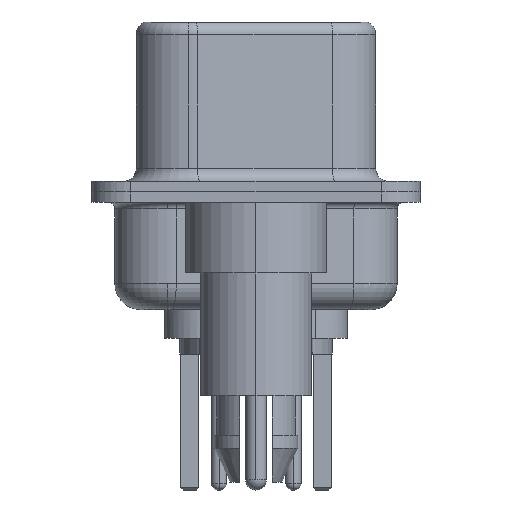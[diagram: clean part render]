
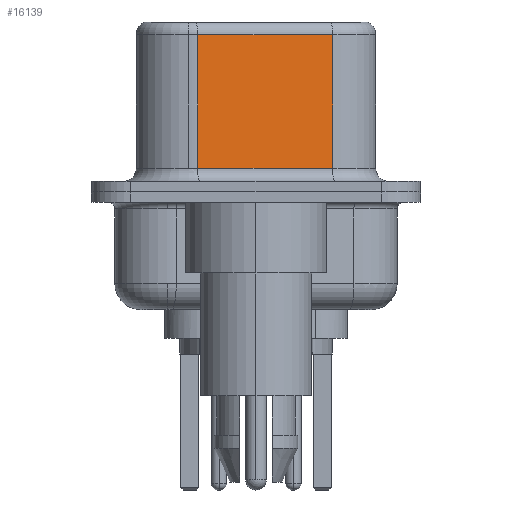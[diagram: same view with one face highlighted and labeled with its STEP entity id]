
A CAD part, left-side view. The second image highlights one B-rep face of the part: STEP entity #16139.
In plain terms, the highlighted planar face has unit normal (-0.985, -0.174, 0).
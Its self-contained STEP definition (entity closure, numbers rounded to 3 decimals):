
#51 = CARTESIAN_POINT ( 'NONE',  ( 4.58, -2.927, 6.02 ) ) ;
#411 = AXIS2_PLACEMENT_3D ( 'NONE', #12200, #4198, #13582 ) ;
#556 = VECTOR ( 'NONE', #16919, 1000. ) ;
#986 = CARTESIAN_POINT ( 'NONE',  ( 3.67, 2.233, 6.02 ) ) ;
#1496 = ORIENTED_EDGE ( 'NONE', *, *, #4866, .T. ) ;
#2880 = PLANE ( 'NONE',  #411 ) ;
#3615 = FACE_OUTER_BOUND ( 'NONE', #12085, .T. ) ;
#3982 = CARTESIAN_POINT ( 'NONE',  ( 3.67, 2.233, 6.52 ) ) ;
#4089 = DIRECTION ( 'NONE',  ( 0., 0., -1. ) ) ;
#4198 = DIRECTION ( 'NONE',  ( 0.985, 0.174, 0. ) ) ;
#4596 = LINE ( 'NONE', #51, #556 ) ;
#4689 = EDGE_CURVE ( 'NONE', #16099, #12478, #4596, .T. ) ;
#4760 = CARTESIAN_POINT ( 'NONE',  ( 3.67, 2.233, 0.9 ) ) ;
#4866 = EDGE_CURVE ( 'NONE', #12478, #5117, #14056, .T. ) ;
#5117 = VERTEX_POINT ( 'NONE', #4760 ) ;
#5636 = VECTOR ( 'NONE', #4089, 1000. ) ;
#6155 = EDGE_CURVE ( 'NONE', #5117, #11291, #13352, .T. ) ;
#6260 = VECTOR ( 'NONE', #12339, 1000. ) ;
#7291 = EDGE_CURVE ( 'NONE', #16099, #11291, #17432, .T. ) ;
#8172 = CARTESIAN_POINT ( 'NONE',  ( 4.58, -2.927, 6.02 ) ) ;
#11291 = VERTEX_POINT ( 'NONE', #11631 ) ;
#11466 = CARTESIAN_POINT ( 'NONE',  ( 4.58, -2.927, 6.52 ) ) ;
#11631 = CARTESIAN_POINT ( 'NONE',  ( 4.58, -2.927, 0.9 ) ) ;
#12085 = EDGE_LOOP ( 'NONE', ( #15302, #17098, #1496, #12354 ) ) ;
#12200 = CARTESIAN_POINT ( 'NONE',  ( 4.58, -2.927, 6.52 ) ) ;
#12339 = DIRECTION ( 'NONE',  ( 0.174, -0.985, 0. ) ) ;
#12354 = ORIENTED_EDGE ( 'NONE', *, *, #6155, .T. ) ;
#12478 = VERTEX_POINT ( 'NONE', #986 ) ;
#13352 = LINE ( 'NONE', #13597, #6260 ) ;
#13582 = DIRECTION ( 'NONE',  ( -0.174, 0.985, 0. ) ) ;
#13597 = CARTESIAN_POINT ( 'NONE',  ( 4.58, -2.927, 0.9 ) ) ;
#13762 = VECTOR ( 'NONE', #16857, 1000. ) ;
#14056 = LINE ( 'NONE', #3982, #5636 ) ;
#15302 = ORIENTED_EDGE ( 'NONE', *, *, #7291, .F. ) ;
#16099 = VERTEX_POINT ( 'NONE', #8172 ) ;
#16139 = ADVANCED_FACE ( 'NONE', ( #3615 ), #2880, .F. ) ;
#16857 = DIRECTION ( 'NONE',  ( 0., 0., -1. ) ) ;
#16919 = DIRECTION ( 'NONE',  ( -0.174, 0.985, 0. ) ) ;
#17098 = ORIENTED_EDGE ( 'NONE', *, *, #4689, .T. ) ;
#17432 = LINE ( 'NONE', #11466, #13762 ) ;
